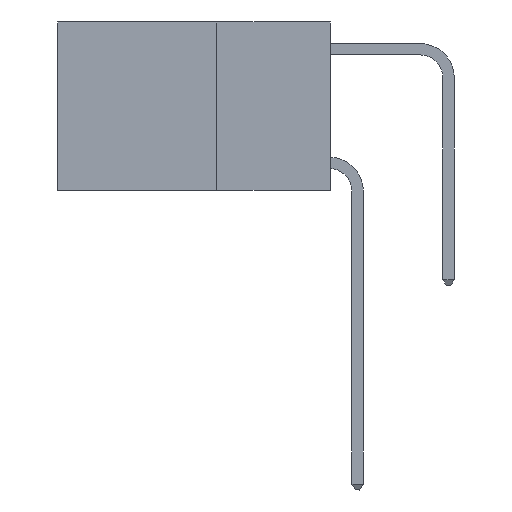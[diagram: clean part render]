
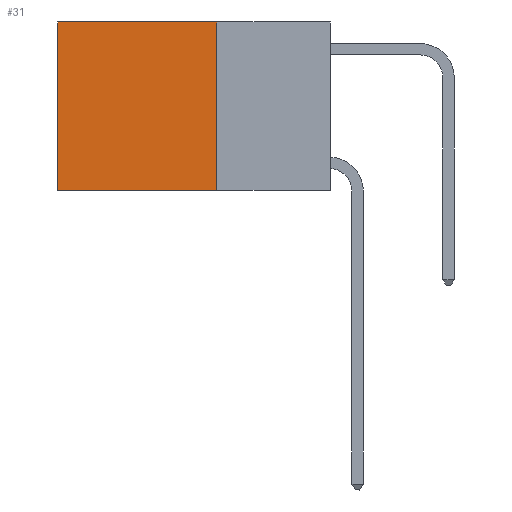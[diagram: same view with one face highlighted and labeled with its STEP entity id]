
A CAD part, left-side view. The second image highlights one B-rep face of the part: STEP entity #31.
In plain terms, the highlighted planar face has unit normal (-1, 0, 0).
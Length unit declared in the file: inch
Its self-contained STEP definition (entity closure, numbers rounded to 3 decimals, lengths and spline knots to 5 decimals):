
#31 = ADVANCED_FACE ( 'NONE', ( #9002 ), #1603, .F. ) ;
#133 = DIRECTION ( 'NONE',  ( 0., 0., -1. ) ) ;
#513 = DIRECTION ( 'NONE',  ( 1., 0., 0. ) ) ;
#1540 = CARTESIAN_POINT ( 'NONE',  ( 0.2625, 0.25, 0. ) ) ;
#1603 = PLANE ( 'NONE',  #19457 ) ;
#1909 = VECTOR ( 'NONE', #9965, 39.37008 ) ;
#2422 = CARTESIAN_POINT ( 'NONE',  ( 0.2625, 0.6, 0. ) ) ;
#3375 = VECTOR ( 'NONE', #10625, 39.37008 ) ;
#4058 = EDGE_CURVE ( 'NONE', #13786, #13139, #14153, .T. ) ;
#5874 = EDGE_CURVE ( 'NONE', #12284, #13139, #7352, .T. ) ;
#7309 = ORIENTED_EDGE ( 'NONE', *, *, #5874, .T. ) ;
#7352 = LINE ( 'NONE', #14132, #1909 ) ;
#8522 = DIRECTION ( 'NONE',  ( 0., 1., 0. ) ) ;
#9002 = FACE_OUTER_BOUND ( 'NONE', #19234, .T. ) ;
#9637 = VECTOR ( 'NONE', #9904, 39.37008 ) ;
#9904 = DIRECTION ( 'NONE',  ( 0., 1., 0. ) ) ;
#9964 = VERTEX_POINT ( 'NONE', #15357 ) ;
#9965 = DIRECTION ( 'NONE',  ( 0., 0., -1. ) ) ;
#10373 = CARTESIAN_POINT ( 'NONE',  ( 0.2625, 0.25, -0.37 ) ) ;
#10625 = DIRECTION ( 'NONE',  ( 0., 0., -1. ) ) ;
#10777 = EDGE_CURVE ( 'NONE', #9964, #12284, #15591, .T. ) ;
#12206 = ORIENTED_EDGE ( 'NONE', *, *, #16479, .F. ) ;
#12284 = VERTEX_POINT ( 'NONE', #2422 ) ;
#13139 = VERTEX_POINT ( 'NONE', #24397 ) ;
#13786 = VERTEX_POINT ( 'NONE', #10373 ) ;
#14132 = CARTESIAN_POINT ( 'NONE',  ( 0.2625, 0.6, 0. ) ) ;
#14153 = LINE ( 'NONE', #20482, #24817 ) ;
#15357 = CARTESIAN_POINT ( 'NONE',  ( 0.2625, 0.25, 0. ) ) ;
#15591 = LINE ( 'NONE', #19826, #9637 ) ;
#16479 = EDGE_CURVE ( 'NONE', #9964, #13786, #18812, .T. ) ;
#16562 = CARTESIAN_POINT ( 'NONE',  ( 0.2625, 0.25, 0. ) ) ;
#18812 = LINE ( 'NONE', #16562, #3375 ) ;
#19234 = EDGE_LOOP ( 'NONE', ( #7309, #20491, #12206, #22466 ) ) ;
#19457 = AXIS2_PLACEMENT_3D ( 'NONE', #1540, #513, #133 ) ;
#19826 = CARTESIAN_POINT ( 'NONE',  ( 0.2625, 0.25, 0. ) ) ;
#20482 = CARTESIAN_POINT ( 'NONE',  ( 0.2625, 0.25, -0.37 ) ) ;
#20491 = ORIENTED_EDGE ( 'NONE', *, *, #4058, .F. ) ;
#22466 = ORIENTED_EDGE ( 'NONE', *, *, #10777, .T. ) ;
#24397 = CARTESIAN_POINT ( 'NONE',  ( 0.2625, 0.6, -0.37 ) ) ;
#24817 = VECTOR ( 'NONE', #8522, 39.37008 ) ;
